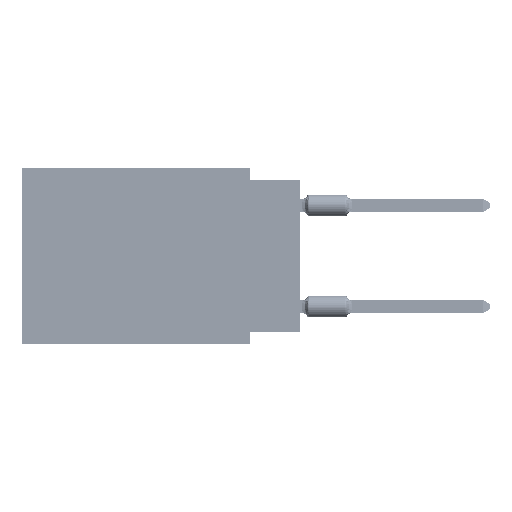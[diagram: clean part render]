
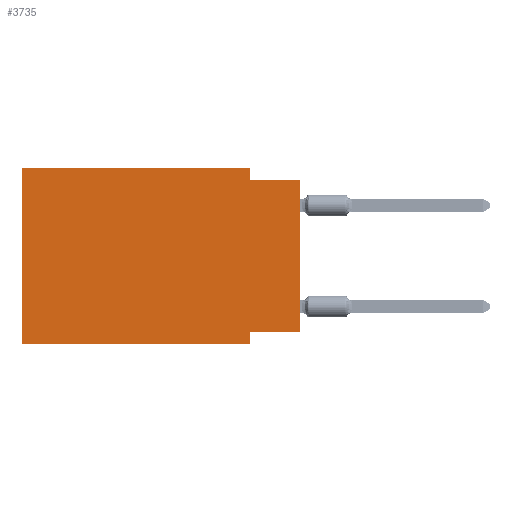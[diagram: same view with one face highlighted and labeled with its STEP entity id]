
A CAD part, left-side view. The second image highlights one B-rep face of the part: STEP entity #3735.
In plain terms, the highlighted planar face has unit normal (-1, 0, 0).
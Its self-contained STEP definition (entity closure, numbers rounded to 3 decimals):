
#971 = CARTESIAN_POINT ( 'NONE',  ( 0., 2.54, -8.89 ) ) ;
#2743 = CARTESIAN_POINT ( 'NONE',  ( 0., 2.54, -0.635 ) ) ;
#3735 = ADVANCED_FACE ( 'NONE', ( #89620 ), #60477, .F. ) ;
#4701 = CARTESIAN_POINT ( 'NONE',  ( 0., 0., -8.255 ) ) ;
#7916 = EDGE_CURVE ( 'NONE', #104189, #99991, #89797, .T. ) ;
#9311 = VERTEX_POINT ( 'NONE', #4701 ) ;
#13687 = DIRECTION ( 'NONE',  ( 0., 0., -1. ) ) ;
#15899 = EDGE_CURVE ( 'NONE', #113803, #35621, #91568, .T. ) ;
#17967 = DIRECTION ( 'NONE',  ( 0., -1., 0. ) ) ;
#18155 = DIRECTION ( 'NONE',  ( 0., 0., -1. ) ) ;
#22154 = VECTOR ( 'NONE', #72119, 1000. ) ;
#26749 = CARTESIAN_POINT ( 'NONE',  ( 0., 0., 0. ) ) ;
#27261 = LINE ( 'NONE', #101403, #87014 ) ;
#28289 = CARTESIAN_POINT ( 'NONE',  ( 0., 0., -0.635 ) ) ;
#30088 = CARTESIAN_POINT ( 'NONE',  ( 0., 2.54, -8.255 ) ) ;
#31933 = DIRECTION ( 'NONE',  ( 1., 0., 0. ) ) ;
#33315 = CARTESIAN_POINT ( 'NONE',  ( 0., 13.97, 0. ) ) ;
#33871 = CARTESIAN_POINT ( 'NONE',  ( 0., 2.54, 0. ) ) ;
#34016 = CARTESIAN_POINT ( 'NONE',  ( 0., 0., -0.635 ) ) ;
#34642 = LINE ( 'NONE', #26749, #60561 ) ;
#35211 = EDGE_CURVE ( 'NONE', #37967, #35621, #27261, .T. ) ;
#35621 = VERTEX_POINT ( 'NONE', #971 ) ;
#36084 = ORIENTED_EDGE ( 'NONE', *, *, #112301, .T. ) ;
#36188 = CARTESIAN_POINT ( 'NONE',  ( 0., 13.97, 0. ) ) ;
#37384 = LINE ( 'NONE', #36188, #70361 ) ;
#37749 = EDGE_CURVE ( 'NONE', #99991, #79138, #55052, .T. ) ;
#37967 = VERTEX_POINT ( 'NONE', #30088 ) ;
#38326 = VECTOR ( 'NONE', #118293, 1000. ) ;
#41945 = ORIENTED_EDGE ( 'NONE', *, *, #93405, .F. ) ;
#43519 = CARTESIAN_POINT ( 'NONE',  ( 0., 13.97, 0. ) ) ;
#46573 = ORIENTED_EDGE ( 'NONE', *, *, #7916, .F. ) ;
#50855 = LINE ( 'NONE', #43519, #38326 ) ;
#51161 = AXIS2_PLACEMENT_3D ( 'NONE', #117009, #31933, #13687 ) ;
#52265 = ORIENTED_EDGE ( 'NONE', *, *, #55287, .F. ) ;
#53927 = DIRECTION ( 'NONE',  ( 0., 0., -1. ) ) ;
#55052 = LINE ( 'NONE', #28289, #71612 ) ;
#55287 = EDGE_CURVE ( 'NONE', #88305, #104189, #37384, .T. ) ;
#60477 = PLANE ( 'NONE',  #51161 ) ;
#60561 = VECTOR ( 'NONE', #119769, 1000. ) ;
#61898 = CARTESIAN_POINT ( 'NONE',  ( 0., 13.97, -8.89 ) ) ;
#63537 = DIRECTION ( 'NONE',  ( 0., 1., 0. ) ) ;
#64863 = EDGE_LOOP ( 'NONE', ( #36084, #73905, #46573, #52265, #41945, #76481, #95777, #109856 ) ) ;
#65369 = DIRECTION ( 'NONE',  ( 0., -1., 0. ) ) ;
#70361 = VECTOR ( 'NONE', #17967, 1000. ) ;
#71612 = VECTOR ( 'NONE', #65369, 1000. ) ;
#72119 = DIRECTION ( 'NONE',  ( 0., -1., 0. ) ) ;
#73905 = ORIENTED_EDGE ( 'NONE', *, *, #37749, .F. ) ;
#73913 = CARTESIAN_POINT ( 'NONE',  ( 0., 13.97, -8.89 ) ) ;
#76481 = ORIENTED_EDGE ( 'NONE', *, *, #15899, .T. ) ;
#79138 = VERTEX_POINT ( 'NONE', #34016 ) ;
#87014 = VECTOR ( 'NONE', #18155, 1000. ) ;
#88305 = VERTEX_POINT ( 'NONE', #33315 ) ;
#89620 = FACE_OUTER_BOUND ( 'NONE', #64863, .T. ) ;
#89797 = LINE ( 'NONE', #33871, #104017 ) ;
#91568 = LINE ( 'NONE', #73913, #22154 ) ;
#93405 = EDGE_CURVE ( 'NONE', #113803, #88305, #50855, .T. ) ;
#95777 = ORIENTED_EDGE ( 'NONE', *, *, #35211, .F. ) ;
#99991 = VERTEX_POINT ( 'NONE', #2743 ) ;
#101403 = CARTESIAN_POINT ( 'NONE',  ( 0., 2.54, -8.89 ) ) ;
#104017 = VECTOR ( 'NONE', #53927, 1000. ) ;
#104189 = VERTEX_POINT ( 'NONE', #119431 ) ;
#108544 = LINE ( 'NONE', #109141, #110104 ) ;
#109141 = CARTESIAN_POINT ( 'NONE',  ( 0., 0., -8.255 ) ) ;
#109856 = ORIENTED_EDGE ( 'NONE', *, *, #119492, .F. ) ;
#110104 = VECTOR ( 'NONE', #63537, 1000. ) ;
#112301 = EDGE_CURVE ( 'NONE', #9311, #79138, #34642, .T. ) ;
#113803 = VERTEX_POINT ( 'NONE', #61898 ) ;
#117009 = CARTESIAN_POINT ( 'NONE',  ( 0., 13.97, 0. ) ) ;
#118293 = DIRECTION ( 'NONE',  ( 0., 0., 1. ) ) ;
#119431 = CARTESIAN_POINT ( 'NONE',  ( 0., 2.54, 0. ) ) ;
#119492 = EDGE_CURVE ( 'NONE', #9311, #37967, #108544, .T. ) ;
#119769 = DIRECTION ( 'NONE',  ( 0., 0., 1. ) ) ;
